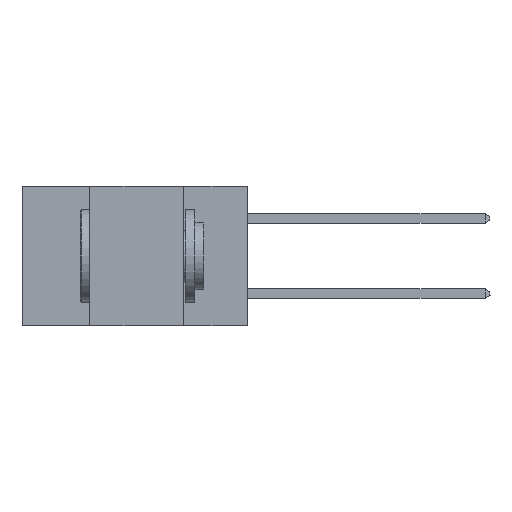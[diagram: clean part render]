
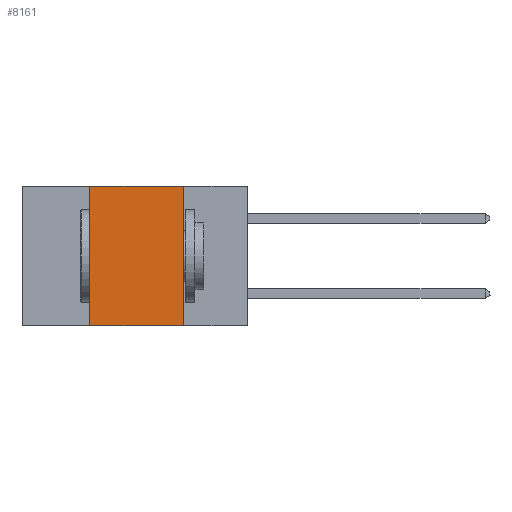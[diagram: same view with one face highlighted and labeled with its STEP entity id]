
A CAD part, left-side view. The second image highlights one B-rep face of the part: STEP entity #8161.
In plain terms, the highlighted planar face has unit normal (-1, 0, 0).
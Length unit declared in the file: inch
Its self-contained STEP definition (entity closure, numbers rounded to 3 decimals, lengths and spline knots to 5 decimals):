
#2290 = CARTESIAN_POINT ( 'NONE',  ( 0., 0.6, 0. ) ) ;
#3415 = FACE_OUTER_BOUND ( 'NONE', #19616, .T. ) ;
#4857 = LINE ( 'NONE', #31180, #30201 ) ;
#5298 = ORIENTED_EDGE ( 'NONE', *, *, #23373, .F. ) ;
#6874 = LINE ( 'NONE', #8714, #12838 ) ;
#6901 = ORIENTED_EDGE ( 'NONE', *, *, #24700, .F. ) ;
#7610 = AXIS2_PLACEMENT_3D ( 'NONE', #2290, #27779, #12619 ) ;
#7941 = VERTEX_POINT ( 'NONE', #19287 ) ;
#8161 = ADVANCED_FACE ( 'NONE', ( #3415 ), #25253, .F. ) ;
#8412 = CARTESIAN_POINT ( 'NONE',  ( 0., 0.6, -0.37 ) ) ;
#8714 = CARTESIAN_POINT ( 'NONE',  ( 0., 0.42, 0. ) ) ;
#9600 = VERTEX_POINT ( 'NONE', #28236 ) ;
#10941 = LINE ( 'NONE', #31694, #22847 ) ;
#10953 = VERTEX_POINT ( 'NONE', #12064 ) ;
#12064 = CARTESIAN_POINT ( 'NONE',  ( 0., 0.42, -0.37 ) ) ;
#12619 = DIRECTION ( 'NONE',  ( 0., 0., -1. ) ) ;
#12838 = VECTOR ( 'NONE', #28925, 39.37008 ) ;
#16571 = DIRECTION ( 'NONE',  ( 0., -1., 0. ) ) ;
#17061 = VECTOR ( 'NONE', #31035, 39.37008 ) ;
#19287 = CARTESIAN_POINT ( 'NONE',  ( 0., 0.17, -0.37 ) ) ;
#19613 = EDGE_CURVE ( 'NONE', #10953, #27935, #6874, .T. ) ;
#19616 = EDGE_LOOP ( 'NONE', ( #6901, #5298, #24763, #25146 ) ) ;
#20478 = CARTESIAN_POINT ( 'NONE',  ( 0., 0.42, 0. ) ) ;
#22847 = VECTOR ( 'NONE', #16571, 39.37008 ) ;
#23373 = EDGE_CURVE ( 'NONE', #27935, #9600, #10941, .T. ) ;
#24700 = EDGE_CURVE ( 'NONE', #9600, #7941, #4857, .T. ) ;
#24763 = ORIENTED_EDGE ( 'NONE', *, *, #19613, .F. ) ;
#25146 = ORIENTED_EDGE ( 'NONE', *, *, #31472, .T. ) ;
#25253 = PLANE ( 'NONE',  #7610 ) ;
#27779 = DIRECTION ( 'NONE',  ( 1., 0., 0. ) ) ;
#27935 = VERTEX_POINT ( 'NONE', #20478 ) ;
#28236 = CARTESIAN_POINT ( 'NONE',  ( 0., 0.17, 0. ) ) ;
#28925 = DIRECTION ( 'NONE',  ( 0., 0., 1. ) ) ;
#30201 = VECTOR ( 'NONE', #31401, 39.37008 ) ;
#30498 = LINE ( 'NONE', #8412, #17061 ) ;
#31035 = DIRECTION ( 'NONE',  ( 0., -1., 0. ) ) ;
#31180 = CARTESIAN_POINT ( 'NONE',  ( 0., 0.17, 0. ) ) ;
#31401 = DIRECTION ( 'NONE',  ( 0., 0., -1. ) ) ;
#31472 = EDGE_CURVE ( 'NONE', #10953, #7941, #30498, .T. ) ;
#31694 = CARTESIAN_POINT ( 'NONE',  ( 0., 0.6, 0. ) ) ;
